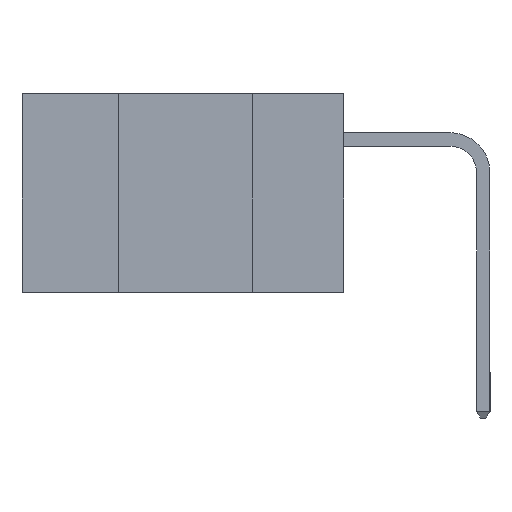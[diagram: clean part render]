
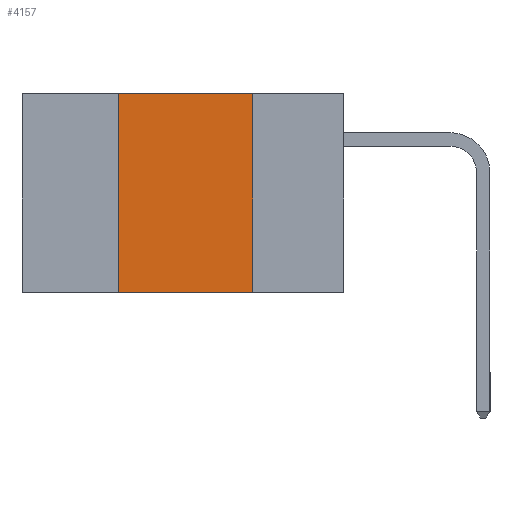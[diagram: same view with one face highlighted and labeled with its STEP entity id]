
A CAD part, left-side view. The second image highlights one B-rep face of the part: STEP entity #4157.
In plain terms, the highlighted planar face has unit normal (-1, 0, 0).
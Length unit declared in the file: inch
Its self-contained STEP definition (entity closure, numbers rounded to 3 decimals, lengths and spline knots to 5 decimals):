
#365 = EDGE_CURVE ( 'NONE', #6659, #4899, #19245, .T. ) ;
#957 = CARTESIAN_POINT ( 'NONE',  ( 0., 0.17, 0. ) ) ;
#1145 = DIRECTION ( 'NONE',  ( 0., -1., 0. ) ) ;
#1181 = ORIENTED_EDGE ( 'NONE', *, *, #2004, .T. ) ;
#1509 = DIRECTION ( 'NONE',  ( 1., 0., 0. ) ) ;
#2004 = EDGE_CURVE ( 'NONE', #17634, #16989, #15195, .T. ) ;
#2852 = CARTESIAN_POINT ( 'NONE',  ( 0., 0.6, -0.37 ) ) ;
#2860 = VECTOR ( 'NONE', #1145, 39.37008 ) ;
#4157 = ADVANCED_FACE ( 'NONE', ( #15866 ), #17093, .F. ) ;
#4899 = VERTEX_POINT ( 'NONE', #957 ) ;
#5083 = DIRECTION ( 'NONE',  ( 0., 0., 1. ) ) ;
#5460 = LINE ( 'NONE', #17401, #15569 ) ;
#6659 = VERTEX_POINT ( 'NONE', #10990 ) ;
#6998 = CARTESIAN_POINT ( 'NONE',  ( 0., 0.6, 0. ) ) ;
#8601 = EDGE_CURVE ( 'NONE', #17634, #6659, #14219, .T. ) ;
#8652 = DIRECTION ( 'NONE',  ( 0., 0., -1. ) ) ;
#8850 = EDGE_LOOP ( 'NONE', ( #16355, #19058, #13644, #1181 ) ) ;
#9046 = EDGE_CURVE ( 'NONE', #4899, #16989, #5460, .T. ) ;
#9838 = DIRECTION ( 'NONE',  ( 0., 0., -1. ) ) ;
#10874 = CARTESIAN_POINT ( 'NONE',  ( 0., 0.6, 0. ) ) ;
#10990 = CARTESIAN_POINT ( 'NONE',  ( 0., 0.42, 0. ) ) ;
#12277 = AXIS2_PLACEMENT_3D ( 'NONE', #10874, #1509, #9838 ) ;
#12715 = CARTESIAN_POINT ( 'NONE',  ( 0., 0.42, -0.37 ) ) ;
#12812 = CARTESIAN_POINT ( 'NONE',  ( 0., 0.42, -0.37 ) ) ;
#12986 = VECTOR ( 'NONE', #5083, 39.37008 ) ;
#13031 = DIRECTION ( 'NONE',  ( 0., -1., 0. ) ) ;
#13644 = ORIENTED_EDGE ( 'NONE', *, *, #8601, .F. ) ;
#14219 = LINE ( 'NONE', #12715, #12986 ) ;
#15195 = LINE ( 'NONE', #2852, #16832 ) ;
#15569 = VECTOR ( 'NONE', #8652, 39.37008 ) ;
#15866 = FACE_OUTER_BOUND ( 'NONE', #8850, .T. ) ;
#16355 = ORIENTED_EDGE ( 'NONE', *, *, #9046, .F. ) ;
#16832 = VECTOR ( 'NONE', #13031, 39.37008 ) ;
#16989 = VERTEX_POINT ( 'NONE', #19480 ) ;
#17093 = PLANE ( 'NONE',  #12277 ) ;
#17401 = CARTESIAN_POINT ( 'NONE',  ( 0., 0.17, -0.37 ) ) ;
#17634 = VERTEX_POINT ( 'NONE', #12812 ) ;
#19058 = ORIENTED_EDGE ( 'NONE', *, *, #365, .F. ) ;
#19245 = LINE ( 'NONE', #6998, #2860 ) ;
#19480 = CARTESIAN_POINT ( 'NONE',  ( 0., 0.17, -0.37 ) ) ;
